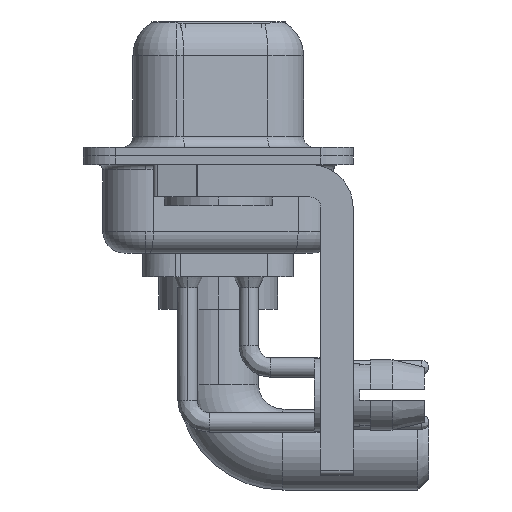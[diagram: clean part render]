
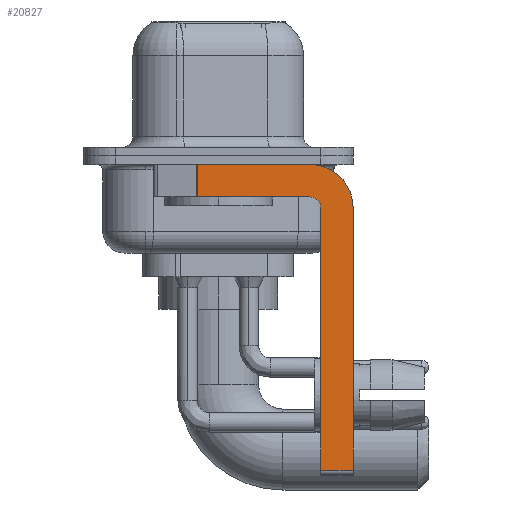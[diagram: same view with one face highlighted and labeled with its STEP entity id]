
A CAD part, left-side view. The second image highlights one B-rep face of the part: STEP entity #20827.
In plain terms, the highlighted planar face has unit normal (-1, 0, 0).
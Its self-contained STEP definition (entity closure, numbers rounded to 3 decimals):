
#56 = VERTEX_POINT ( 'NONE', #12256 ) ;
#211 = LINE ( 'NONE', #18001, #14365 ) ;
#638 = VERTEX_POINT ( 'NONE', #6301 ) ;
#673 = LINE ( 'NONE', #15085, #5503 ) ;
#876 = ORIENTED_EDGE ( 'NONE', *, *, #9366, .F. ) ;
#1421 = DIRECTION ( 'NONE',  ( 1., 0., 0. ) ) ;
#1668 = DIRECTION ( 'NONE',  ( 0., 0., -1. ) ) ;
#1677 = VECTOR ( 'NONE', #14837, 1000. ) ;
#2187 = CARTESIAN_POINT ( 'NONE',  ( -2.9, -4.25, -1.9 ) ) ;
#3053 = VECTOR ( 'NONE', #16039, 1000. ) ;
#3192 = CARTESIAN_POINT ( 'NONE',  ( -2.9, -4.25, -2.4 ) ) ;
#4089 = DIRECTION ( 'NONE',  ( 0., 0., 1. ) ) ;
#4196 = VERTEX_POINT ( 'NONE', #15575 ) ;
#4605 = ORIENTED_EDGE ( 'NONE', *, *, #7669, .F. ) ;
#5212 = EDGE_CURVE ( 'NONE', #16345, #6946, #673, .T. ) ;
#5294 = ORIENTED_EDGE ( 'NONE', *, *, #13506, .F. ) ;
#5503 = VECTOR ( 'NONE', #9041, 1000. ) ;
#5560 = ORIENTED_EDGE ( 'NONE', *, *, #19612, .F. ) ;
#5577 = LINE ( 'NONE', #15379, #8149 ) ;
#5927 = DIRECTION ( 'NONE',  ( 0., 0., -1. ) ) ;
#5934 = DIRECTION ( 'NONE',  ( 0., 0., -1. ) ) ;
#6026 = PLANE ( 'NONE',  #9145 ) ;
#6301 = CARTESIAN_POINT ( 'NONE',  ( -2.9, -4.75, -2.4 ) ) ;
#6323 = CARTESIAN_POINT ( 'NONE',  ( -2.9, -4.25, -14.55 ) ) ;
#6886 = CIRCLE ( 'NONE', #16662, 0.5 ) ;
#6946 = VERTEX_POINT ( 'NONE', #7319 ) ;
#7047 = DIRECTION ( 'NONE',  ( 0., -1., 0. ) ) ;
#7319 = CARTESIAN_POINT ( 'NONE',  ( -2.9, 0.978, -1.9 ) ) ;
#7507 = FACE_OUTER_BOUND ( 'NONE', #15061, .T. ) ;
#7609 = CARTESIAN_POINT ( 'NONE',  ( -2.9, -4.25, -0.4 ) ) ;
#7669 = EDGE_CURVE ( 'NONE', #638, #7879, #6886, .T. ) ;
#7879 = VERTEX_POINT ( 'NONE', #16325 ) ;
#8149 = VECTOR ( 'NONE', #7047, 1000. ) ;
#8601 = LINE ( 'NONE', #11758, #16616 ) ;
#9041 = DIRECTION ( 'NONE',  ( 0., 0., -1. ) ) ;
#9145 = AXIS2_PLACEMENT_3D ( 'NONE', #9209, #12683, #5927 ) ;
#9209 = CARTESIAN_POINT ( 'NONE',  ( -2.9, -4.25, -2.4 ) ) ;
#9366 = EDGE_CURVE ( 'NONE', #7879, #6946, #19577, .T. ) ;
#9800 = EDGE_CURVE ( 'NONE', #20774, #4196, #13465, .T. ) ;
#10187 = DIRECTION ( 'NONE',  ( 0., 0., 1. ) ) ;
#10770 = EDGE_CURVE ( 'NONE', #18949, #56, #10776, .T. ) ;
#10776 = LINE ( 'NONE', #6323, #3053 ) ;
#11344 = ORIENTED_EDGE ( 'NONE', *, *, #10770, .T. ) ;
#11758 = CARTESIAN_POINT ( 'NONE',  ( -2.9, -4.75, -14.8 ) ) ;
#12256 = CARTESIAN_POINT ( 'NONE',  ( -2.9, -6.25, -14.55 ) ) ;
#12642 = ORIENTED_EDGE ( 'NONE', *, *, #5212, .T. ) ;
#12683 = DIRECTION ( 'NONE',  ( 1., 0., 0. ) ) ;
#12801 = CARTESIAN_POINT ( 'NONE',  ( -2.9, 0.978, -0.4 ) ) ;
#13465 = CIRCLE ( 'NONE', #18503, 2. ) ;
#13506 = EDGE_CURVE ( 'NONE', #16345, #20774, #5577, .T. ) ;
#14365 = VECTOR ( 'NONE', #1668, 1000. ) ;
#14776 = ORIENTED_EDGE ( 'NONE', *, *, #9800, .F. ) ;
#14837 = DIRECTION ( 'NONE',  ( 0., 1., 0. ) ) ;
#14859 = EDGE_CURVE ( 'NONE', #18949, #638, #8601, .T. ) ;
#15061 = EDGE_LOOP ( 'NONE', ( #5294, #12642, #876, #4605, #15683, #11344, #5560, #14776 ) ) ;
#15085 = CARTESIAN_POINT ( 'NONE',  ( -2.9, 0.978, -1.9 ) ) ;
#15379 = CARTESIAN_POINT ( 'NONE',  ( -2.9, 3., -0.4 ) ) ;
#15575 = CARTESIAN_POINT ( 'NONE',  ( -2.9, -6.25, -2.4 ) ) ;
#15683 = ORIENTED_EDGE ( 'NONE', *, *, #14859, .F. ) ;
#16039 = DIRECTION ( 'NONE',  ( 0., -1., 0. ) ) ;
#16325 = CARTESIAN_POINT ( 'NONE',  ( -2.9, -4.25, -1.9 ) ) ;
#16345 = VERTEX_POINT ( 'NONE', #12801 ) ;
#16492 = CARTESIAN_POINT ( 'NONE',  ( -2.9, -4.75, -14.55 ) ) ;
#16616 = VECTOR ( 'NONE', #10187, 1000. ) ;
#16662 = AXIS2_PLACEMENT_3D ( 'NONE', #18535, #18642, #4089 ) ;
#18001 = CARTESIAN_POINT ( 'NONE',  ( -2.9, -6.25, -2.4 ) ) ;
#18503 = AXIS2_PLACEMENT_3D ( 'NONE', #3192, #1421, #5934 ) ;
#18535 = CARTESIAN_POINT ( 'NONE',  ( -2.9, -4.25, -2.4 ) ) ;
#18642 = DIRECTION ( 'NONE',  ( -1., 0., 0. ) ) ;
#18949 = VERTEX_POINT ( 'NONE', #16492 ) ;
#19577 = LINE ( 'NONE', #2187, #1677 ) ;
#19612 = EDGE_CURVE ( 'NONE', #4196, #56, #211, .T. ) ;
#20774 = VERTEX_POINT ( 'NONE', #7609 ) ;
#20827 = ADVANCED_FACE ( 'NONE', ( #7507 ), #6026, .F. ) ;
